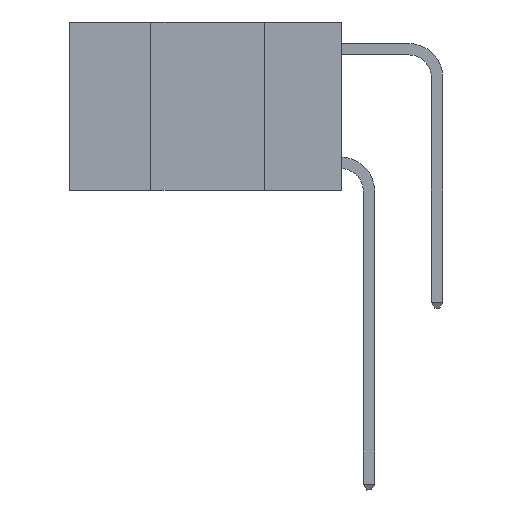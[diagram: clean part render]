
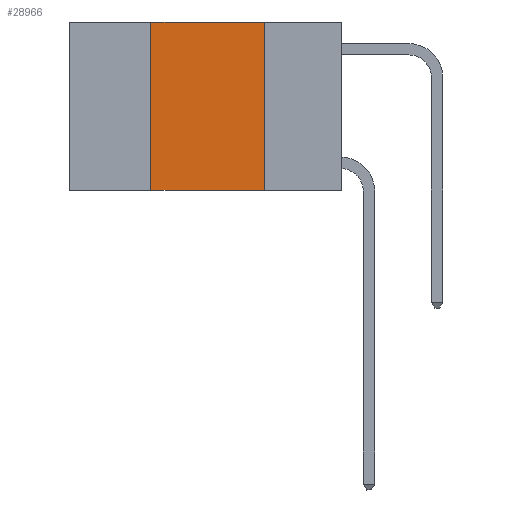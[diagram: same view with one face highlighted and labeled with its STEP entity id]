
A CAD part, left-side view. The second image highlights one B-rep face of the part: STEP entity #28966.
In plain terms, the highlighted planar face has unit normal (-1, 0, 0).
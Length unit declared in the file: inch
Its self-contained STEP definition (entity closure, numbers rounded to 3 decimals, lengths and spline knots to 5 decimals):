
#1127 = EDGE_CURVE ( 'NONE', #9115, #31181, #22698, .T. ) ;
#3026 = DIRECTION ( 'NONE',  ( 0., 0., -1. ) ) ;
#3129 = ORIENTED_EDGE ( 'NONE', *, *, #1127, .F. ) ;
#3188 = CARTESIAN_POINT ( 'NONE',  ( 0., 0.6, 0. ) ) ;
#3314 = CARTESIAN_POINT ( 'NONE',  ( 0., 0.17, 0. ) ) ;
#3437 = LINE ( 'NONE', #16803, #18932 ) ;
#3575 = CARTESIAN_POINT ( 'NONE',  ( 0., 0.6, 0. ) ) ;
#5489 = EDGE_CURVE ( 'NONE', #31181, #33454, #27386, .T. ) ;
#6317 = EDGE_LOOP ( 'NONE', ( #26574, #3129, #22817, #24665 ) ) ;
#7734 = EDGE_CURVE ( 'NONE', #15009, #9115, #34206, .T. ) ;
#9115 = VERTEX_POINT ( 'NONE', #29467 ) ;
#9897 = VECTOR ( 'NONE', #10137, 39.37008 ) ;
#10137 = DIRECTION ( 'NONE',  ( 0., 0., 1. ) ) ;
#13221 = CARTESIAN_POINT ( 'NONE',  ( 0., 0.17, -0.37 ) ) ;
#13560 = DIRECTION ( 'NONE',  ( 1., 0., 0. ) ) ;
#14258 = DIRECTION ( 'NONE',  ( 0., -1., 0. ) ) ;
#15009 = VERTEX_POINT ( 'NONE', #15601 ) ;
#15601 = CARTESIAN_POINT ( 'NONE',  ( 0., 0.42, -0.37 ) ) ;
#16221 = PLANE ( 'NONE',  #23986 ) ;
#16803 = CARTESIAN_POINT ( 'NONE',  ( 0., 0.6, -0.37 ) ) ;
#18424 = CARTESIAN_POINT ( 'NONE',  ( 0., 0.17, 0. ) ) ;
#18719 = DIRECTION ( 'NONE',  ( 0., -1., 0. ) ) ;
#18932 = VECTOR ( 'NONE', #18719, 39.37008 ) ;
#22698 = LINE ( 'NONE', #3575, #27874 ) ;
#22817 = ORIENTED_EDGE ( 'NONE', *, *, #7734, .F. ) ;
#22925 = DIRECTION ( 'NONE',  ( 0., 0., -1. ) ) ;
#23986 = AXIS2_PLACEMENT_3D ( 'NONE', #3188, #13560, #3026 ) ;
#24140 = FACE_OUTER_BOUND ( 'NONE', #6317, .T. ) ;
#24665 = ORIENTED_EDGE ( 'NONE', *, *, #29803, .T. ) ;
#25538 = VECTOR ( 'NONE', #22925, 39.37008 ) ;
#26574 = ORIENTED_EDGE ( 'NONE', *, *, #5489, .F. ) ;
#27386 = LINE ( 'NONE', #3314, #25538 ) ;
#27874 = VECTOR ( 'NONE', #14258, 39.37008 ) ;
#28966 = ADVANCED_FACE ( 'NONE', ( #24140 ), #16221, .F. ) ;
#29467 = CARTESIAN_POINT ( 'NONE',  ( 0., 0.42, 0. ) ) ;
#29803 = EDGE_CURVE ( 'NONE', #15009, #33454, #3437, .T. ) ;
#31181 = VERTEX_POINT ( 'NONE', #18424 ) ;
#31218 = CARTESIAN_POINT ( 'NONE',  ( 0., 0.42, 0. ) ) ;
#33454 = VERTEX_POINT ( 'NONE', #13221 ) ;
#34206 = LINE ( 'NONE', #31218, #9897 ) ;
